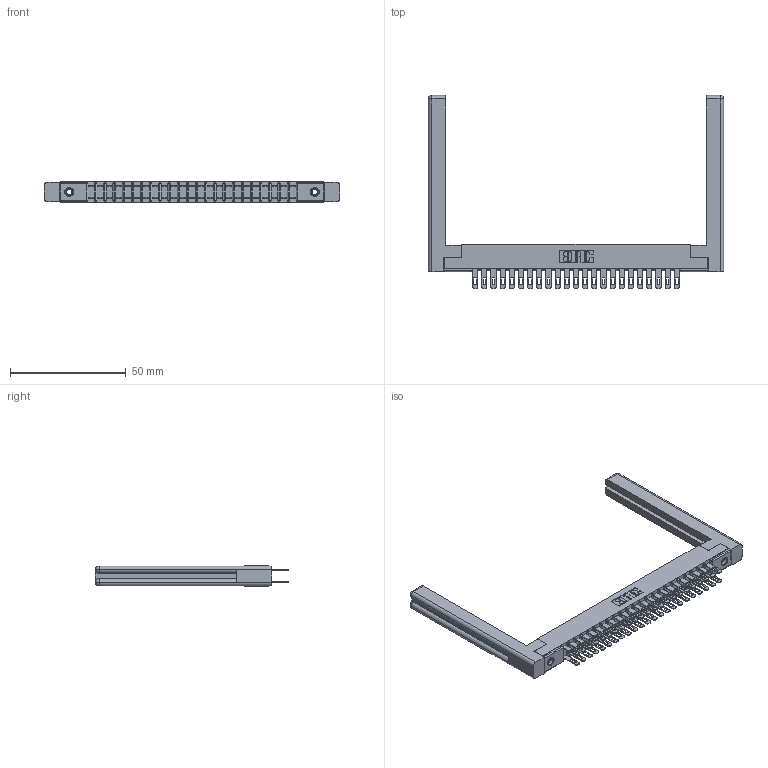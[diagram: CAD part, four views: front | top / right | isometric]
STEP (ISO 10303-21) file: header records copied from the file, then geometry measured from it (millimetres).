
FILE_DESCRIPTION (( 'STEP AP203' ), '1' );
FILE_NAME ('307-046-500-258.STEP', '2019-09-06T08:22:27', ( '' ), ( '' ), 'SwSTEP 2.0', 'SolidWorks 2016', '' );
FILE_SCHEMA (( 'CONFIG_CONTROL_DESIGN' ));
Length unit declared in the file: inch
Products named in the file (5): 307-046-500-258; 345-250-001_345-250-001-102; 307-290-001_500; 307 Part_.156 Dia Mounting Holes; 307-220-058
Assembly tree (51 placements, depth 2):
  307-046-500-258
    307 Part_.156 Dia Mounting Holes
    307-290-001_500  x46
    307-220-058  x2
    345-250-001_345-250-001-102  x2
Bounding box: 127.76 x 83.49 x 8.71 mm (x, y, z)
Volume: 16175.3 mm3; surface area: 20865.9 mm2
Topology: 51 solids, 51 shells, 2400 faces, 6657 edges, 4298 vertices
Faces by surface type: plane 1534, cylinder 794, sphere 48, torus 12, cone 12
Entity records: 25403 total; most frequent: CARTESIAN_POINT 4178, ORIENTED_EDGE 4080, DIRECTION 4060, EDGE_CURVE 2040, LINE 1552, VECTOR 1552, VERTEX_POINT 1318, AXIS2_PLACEMENT_3D 1254
